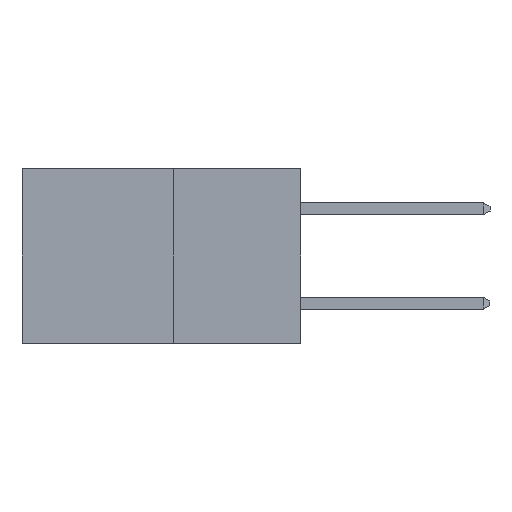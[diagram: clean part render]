
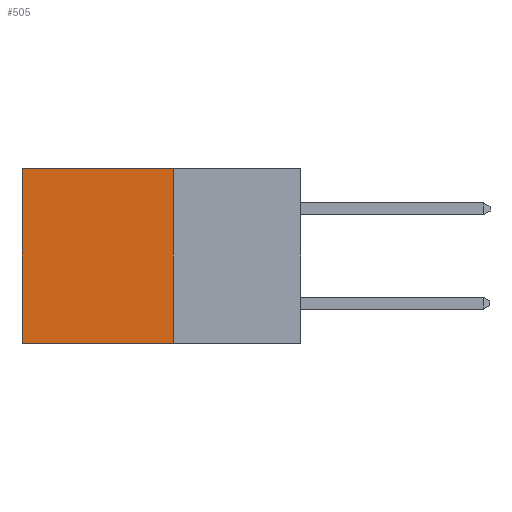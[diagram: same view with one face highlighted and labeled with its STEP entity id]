
A CAD part, left-side view. The second image highlights one B-rep face of the part: STEP entity #505.
In plain terms, the highlighted planar face has unit normal (-1, 0, 0).
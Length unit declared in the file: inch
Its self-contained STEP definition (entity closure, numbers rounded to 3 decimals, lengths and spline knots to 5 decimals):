
#298 = CARTESIAN_POINT ( 'NONE',  ( 0.277, 0.59, -0.37 ) ) ;
#505 = ADVANCED_FACE ( 'NONE', ( #1094 ), #2270, .F. ) ;
#667 = VERTEX_POINT ( 'NONE', #6812 ) ;
#808 = VERTEX_POINT ( 'NONE', #876 ) ;
#876 = CARTESIAN_POINT ( 'NONE',  ( 0.277, 0.27, 0. ) ) ;
#938 = DIRECTION ( 'NONE',  ( 0., 1., 0. ) ) ;
#964 = CARTESIAN_POINT ( 'NONE',  ( 0.277, 0.27, -0.37 ) ) ;
#982 = EDGE_CURVE ( 'NONE', #667, #8677, #4610, .T. ) ;
#1094 = FACE_OUTER_BOUND ( 'NONE', #6736, .T. ) ;
#1364 = DIRECTION ( 'NONE',  ( 0., 1., 0. ) ) ;
#1426 = LINE ( 'NONE', #5932, #1654 ) ;
#1602 = CARTESIAN_POINT ( 'NONE',  ( 0.277, 0.27, -0.37 ) ) ;
#1623 = DIRECTION ( 'NONE',  ( 0., 0., -1. ) ) ;
#1654 = VECTOR ( 'NONE', #3161, 39.37008 ) ;
#1755 = DIRECTION ( 'NONE',  ( 0., 0., -1. ) ) ;
#2270 = PLANE ( 'NONE',  #7734 ) ;
#2386 = VERTEX_POINT ( 'NONE', #3190 ) ;
#2445 = VECTOR ( 'NONE', #1364, 39.37008 ) ;
#2794 = CARTESIAN_POINT ( 'NONE',  ( 0.277, 0.27, 0. ) ) ;
#2990 = ORIENTED_EDGE ( 'NONE', *, *, #8044, .F. ) ;
#3013 = DIRECTION ( 'NONE',  ( 1., 0., 0. ) ) ;
#3161 = DIRECTION ( 'NONE',  ( 0., 0., -1. ) ) ;
#3190 = CARTESIAN_POINT ( 'NONE',  ( 0.277, 0.27, -0.37 ) ) ;
#3454 = EDGE_CURVE ( 'NONE', #2386, #8677, #4922, .T. ) ;
#4080 = ORIENTED_EDGE ( 'NONE', *, *, #982, .T. ) ;
#4515 = LINE ( 'NONE', #2794, #2445 ) ;
#4610 = LINE ( 'NONE', #298, #6240 ) ;
#4922 = LINE ( 'NONE', #964, #6969 ) ;
#5932 = CARTESIAN_POINT ( 'NONE',  ( 0.277, 0.27, -0.37 ) ) ;
#6240 = VECTOR ( 'NONE', #1623, 39.37008 ) ;
#6736 = EDGE_LOOP ( 'NONE', ( #4080, #8943, #2990, #8120 ) ) ;
#6812 = CARTESIAN_POINT ( 'NONE',  ( 0.277, 0.59, 0. ) ) ;
#6969 = VECTOR ( 'NONE', #938, 39.37008 ) ;
#7647 = EDGE_CURVE ( 'NONE', #808, #667, #4515, .T. ) ;
#7734 = AXIS2_PLACEMENT_3D ( 'NONE', #1602, #3013, #1755 ) ;
#7992 = CARTESIAN_POINT ( 'NONE',  ( 0.277, 0.59, -0.37 ) ) ;
#8044 = EDGE_CURVE ( 'NONE', #808, #2386, #1426, .T. ) ;
#8120 = ORIENTED_EDGE ( 'NONE', *, *, #7647, .T. ) ;
#8677 = VERTEX_POINT ( 'NONE', #7992 ) ;
#8943 = ORIENTED_EDGE ( 'NONE', *, *, #3454, .F. ) ;
